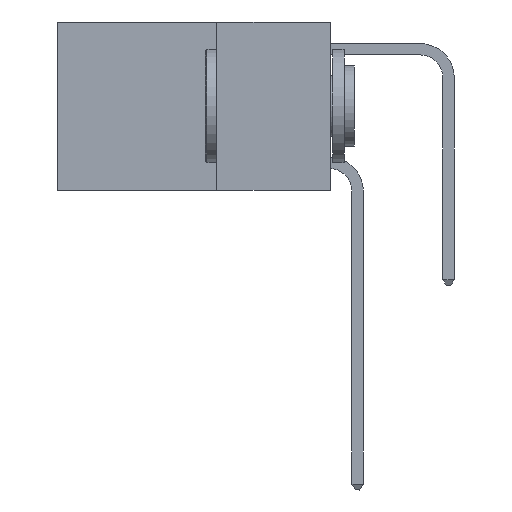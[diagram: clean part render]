
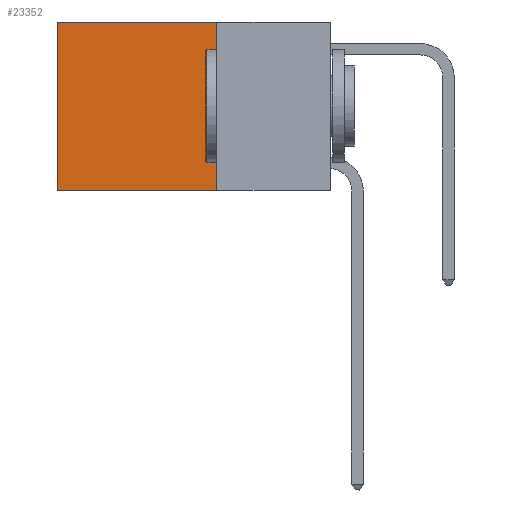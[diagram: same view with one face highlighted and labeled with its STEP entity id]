
A CAD part, left-side view. The second image highlights one B-rep face of the part: STEP entity #23352.
In plain terms, the highlighted planar face has unit normal (-1, 0, 0).
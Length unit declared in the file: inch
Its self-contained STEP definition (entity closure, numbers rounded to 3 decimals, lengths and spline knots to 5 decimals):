
#254 = VERTEX_POINT ( 'NONE', #6021 ) ;
#1359 = ORIENTED_EDGE ( 'NONE', *, *, #26988, .F. ) ;
#2511 = ORIENTED_EDGE ( 'NONE', *, *, #9963, .T. ) ;
#2524 = LINE ( 'NONE', #22976, #11212 ) ;
#2816 = CARTESIAN_POINT ( 'NONE',  ( 0.2625, 0.25, 0. ) ) ;
#4299 = VECTOR ( 'NONE', #24336, 39.37008 ) ;
#5400 = ORIENTED_EDGE ( 'NONE', *, *, #16472, .T. ) ;
#6021 = CARTESIAN_POINT ( 'NONE',  ( 0.2625, 0.25, -0.37 ) ) ;
#6464 = EDGE_CURVE ( 'NONE', #254, #10590, #8688, .T. ) ;
#8688 = LINE ( 'NONE', #15845, #12254 ) ;
#9963 = EDGE_CURVE ( 'NONE', #17712, #12494, #26688, .T. ) ;
#10247 = EDGE_LOOP ( 'NONE', ( #5400, #29748, #1359, #2511 ) ) ;
#10590 = VERTEX_POINT ( 'NONE', #27419 ) ;
#11212 = VECTOR ( 'NONE', #15933, 39.37008 ) ;
#12254 = VECTOR ( 'NONE', #25407, 39.37008 ) ;
#12494 = VERTEX_POINT ( 'NONE', #30292 ) ;
#14016 = VECTOR ( 'NONE', #29326, 39.37008 ) ;
#15830 = DIRECTION ( 'NONE',  ( 0., 0., -1. ) ) ;
#15845 = CARTESIAN_POINT ( 'NONE',  ( 0.2625, 0.25, -0.37 ) ) ;
#15933 = DIRECTION ( 'NONE',  ( 0., 0., -1. ) ) ;
#16142 = DIRECTION ( 'NONE',  ( 1., 0., 0. ) ) ;
#16472 = EDGE_CURVE ( 'NONE', #12494, #10590, #2524, .T. ) ;
#17712 = VERTEX_POINT ( 'NONE', #28326 ) ;
#21157 = PLANE ( 'NONE',  #23365 ) ;
#22254 = LINE ( 'NONE', #22404, #14016 ) ;
#22404 = CARTESIAN_POINT ( 'NONE',  ( 0.2625, 0.25, 0. ) ) ;
#22976 = CARTESIAN_POINT ( 'NONE',  ( 0.2625, 0.6, 0. ) ) ;
#23352 = ADVANCED_FACE ( 'NONE', ( #25867 ), #21157, .F. ) ;
#23365 = AXIS2_PLACEMENT_3D ( 'NONE', #27754, #16142, #15830 ) ;
#24336 = DIRECTION ( 'NONE',  ( 0., 1., 0. ) ) ;
#25407 = DIRECTION ( 'NONE',  ( 0., 1., 0. ) ) ;
#25867 = FACE_OUTER_BOUND ( 'NONE', #10247, .T. ) ;
#26688 = LINE ( 'NONE', #2816, #4299 ) ;
#26988 = EDGE_CURVE ( 'NONE', #17712, #254, #22254, .T. ) ;
#27419 = CARTESIAN_POINT ( 'NONE',  ( 0.2625, 0.6, -0.37 ) ) ;
#27754 = CARTESIAN_POINT ( 'NONE',  ( 0.2625, 0.25, 0. ) ) ;
#28326 = CARTESIAN_POINT ( 'NONE',  ( 0.2625, 0.25, 0. ) ) ;
#29326 = DIRECTION ( 'NONE',  ( 0., 0., -1. ) ) ;
#29748 = ORIENTED_EDGE ( 'NONE', *, *, #6464, .F. ) ;
#30292 = CARTESIAN_POINT ( 'NONE',  ( 0.2625, 0.6, 0. ) ) ;
